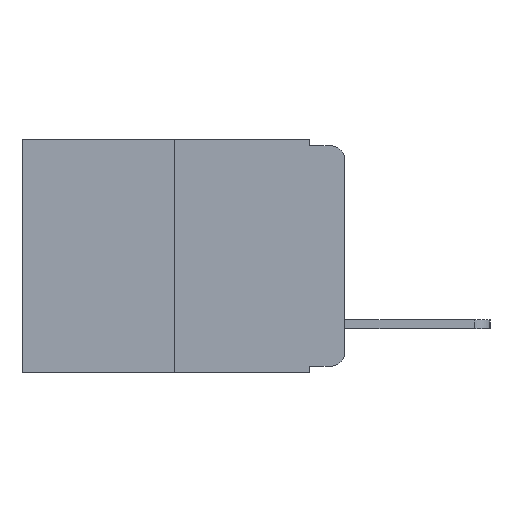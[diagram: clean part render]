
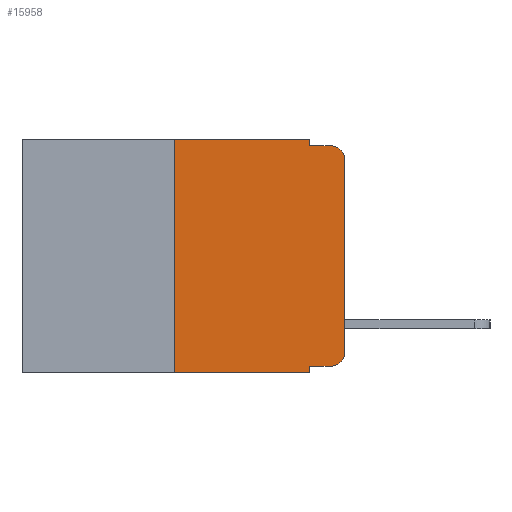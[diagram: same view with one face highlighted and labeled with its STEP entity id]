
A CAD part, left-side view. The second image highlights one B-rep face of the part: STEP entity #15958.
In plain terms, the highlighted planar face has unit normal (-1, 0, 0).
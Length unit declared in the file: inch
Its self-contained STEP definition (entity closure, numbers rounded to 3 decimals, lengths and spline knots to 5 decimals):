
#95 = CARTESIAN_POINT ( 'NONE',  ( 0., 0.25, 0. ) ) ;
#441 = VERTEX_POINT ( 'NONE', #7522 ) ;
#629 = EDGE_CURVE ( 'NONE', #5599, #12527, #10809, .T. ) ;
#1197 = DIRECTION ( 'NONE',  ( 0., -1., 0. ) ) ;
#1220 = VERTEX_POINT ( 'NONE', #19492 ) ;
#1648 = DIRECTION ( 'NONE',  ( 0., 0., -1. ) ) ;
#2439 = VECTOR ( 'NONE', #12449, 39.37008 ) ;
#2592 = CARTESIAN_POINT ( 'NONE',  ( 0., 0.473, 0. ) ) ;
#2681 = VERTEX_POINT ( 'NONE', #3654 ) ;
#2870 = VECTOR ( 'NONE', #18959, 39.37008 ) ;
#2916 = CARTESIAN_POINT ( 'NONE',  ( 0., 0.051, -0.333 ) ) ;
#3638 = CIRCLE ( 'NONE', #15646, 0.02 ) ;
#3654 = CARTESIAN_POINT ( 'NONE',  ( 0., 0.051, -0.333 ) ) ;
#3659 = CARTESIAN_POINT ( 'NONE',  ( 0., 0., 0. ) ) ;
#3790 = DIRECTION ( 'NONE',  ( -1., 0., 0. ) ) ;
#3918 = ORIENTED_EDGE ( 'NONE', *, *, #629, .T. ) ;
#4250 = VECTOR ( 'NONE', #19402, 39.37008 ) ;
#4406 = ORIENTED_EDGE ( 'NONE', *, *, #18420, .T. ) ;
#4427 = EDGE_CURVE ( 'NONE', #5599, #7400, #14295, .T. ) ;
#4751 = CARTESIAN_POINT ( 'NONE',  ( 0., 0.051, -0.01 ) ) ;
#5049 = CARTESIAN_POINT ( 'NONE',  ( 0., 0.473, 0. ) ) ;
#5148 = EDGE_CURVE ( 'NONE', #16173, #11152, #12284, .T. ) ;
#5599 = VERTEX_POINT ( 'NONE', #11612 ) ;
#5987 = CARTESIAN_POINT ( 'NONE',  ( 0., 0.051, 0. ) ) ;
#6458 = VECTOR ( 'NONE', #10842, 39.37008 ) ;
#6759 = VECTOR ( 'NONE', #10499, 39.37008 ) ;
#6897 = LINE ( 'NONE', #2592, #2439 ) ;
#7197 = EDGE_CURVE ( 'NONE', #7400, #18671, #6897, .T. ) ;
#7289 = LINE ( 'NONE', #15903, #2870 ) ;
#7373 = CARTESIAN_POINT ( 'NONE',  ( 0., 0., -0.03 ) ) ;
#7400 = VERTEX_POINT ( 'NONE', #19172 ) ;
#7522 = CARTESIAN_POINT ( 'NONE',  ( 0., 0.02, -0.333 ) ) ;
#7533 = ORIENTED_EDGE ( 'NONE', *, *, #14591, .F. ) ;
#7829 = DIRECTION ( 'NONE',  ( 0., 0., 1. ) ) ;
#8382 = PLANE ( 'NONE',  #8716 ) ;
#8716 = AXIS2_PLACEMENT_3D ( 'NONE', #5049, #11561, #1648 ) ;
#8896 = CARTESIAN_POINT ( 'NONE',  ( 0., 0.051, 0. ) ) ;
#9245 = CARTESIAN_POINT ( 'NONE',  ( 0., 0., -0.313 ) ) ;
#9263 = DIRECTION ( 'NONE',  ( 0., 0., 1. ) ) ;
#9367 = LINE ( 'NONE', #2916, #20849 ) ;
#9461 = CARTESIAN_POINT ( 'NONE',  ( 0., 0.02, -0.313 ) ) ;
#10024 = CARTESIAN_POINT ( 'NONE',  ( 0., 0.051, 0. ) ) ;
#10499 = DIRECTION ( 'NONE',  ( 0., 0., -1. ) ) ;
#10624 = FACE_OUTER_BOUND ( 'NONE', #10813, .T. ) ;
#10809 = LINE ( 'NONE', #17105, #6458 ) ;
#10813 = EDGE_LOOP ( 'NONE', ( #17731, #4406, #10919, #13782, #14993, #13583, #3918, #7533, #17400, #12606 ) ) ;
#10842 = DIRECTION ( 'NONE',  ( 0., -1., 0. ) ) ;
#10919 = ORIENTED_EDGE ( 'NONE', *, *, #17380, .F. ) ;
#11004 = DIRECTION ( 'NONE',  ( 0., 0., -1. ) ) ;
#11014 = EDGE_CURVE ( 'NONE', #18671, #12845, #11101, .T. ) ;
#11101 = LINE ( 'NONE', #8896, #6759 ) ;
#11152 = VERTEX_POINT ( 'NONE', #7373 ) ;
#11405 = EDGE_CURVE ( 'NONE', #441, #16173, #3638, .T. ) ;
#11561 = DIRECTION ( 'NONE',  ( 1., 0., 0. ) ) ;
#11612 = CARTESIAN_POINT ( 'NONE',  ( 0., 0.25, -0.343 ) ) ;
#11808 = VECTOR ( 'NONE', #7829, 39.37008 ) ;
#12284 = LINE ( 'NONE', #3659, #11808 ) ;
#12371 = LINE ( 'NONE', #10024, #4250 ) ;
#12427 = EDGE_CURVE ( 'NONE', #2681, #441, #9367, .T. ) ;
#12449 = DIRECTION ( 'NONE',  ( 0., -1., 0. ) ) ;
#12527 = VERTEX_POINT ( 'NONE', #14508 ) ;
#12606 = ORIENTED_EDGE ( 'NONE', *, *, #11405, .T. ) ;
#12845 = VERTEX_POINT ( 'NONE', #4751 ) ;
#13484 = CARTESIAN_POINT ( 'NONE',  ( 0., 0.02, -0.03 ) ) ;
#13583 = ORIENTED_EDGE ( 'NONE', *, *, #4427, .F. ) ;
#13763 = VECTOR ( 'NONE', #9263, 39.37008 ) ;
#13782 = ORIENTED_EDGE ( 'NONE', *, *, #11014, .F. ) ;
#14295 = LINE ( 'NONE', #95, #13763 ) ;
#14508 = CARTESIAN_POINT ( 'NONE',  ( 0., 0.051, -0.343 ) ) ;
#14591 = EDGE_CURVE ( 'NONE', #2681, #12527, #12371, .T. ) ;
#14993 = ORIENTED_EDGE ( 'NONE', *, *, #7197, .F. ) ;
#15143 = DIRECTION ( 'NONE',  ( 0., 0., -1. ) ) ;
#15646 = AXIS2_PLACEMENT_3D ( 'NONE', #9461, #20406, #11004 ) ;
#15804 = CIRCLE ( 'NONE', #16048, 0.02 ) ;
#15903 = CARTESIAN_POINT ( 'NONE',  ( 0., 0.051, -0.01 ) ) ;
#15958 = ADVANCED_FACE ( 'NONE', ( #10624 ), #8382, .F. ) ;
#16048 = AXIS2_PLACEMENT_3D ( 'NONE', #13484, #3790, #15143 ) ;
#16173 = VERTEX_POINT ( 'NONE', #9245 ) ;
#17105 = CARTESIAN_POINT ( 'NONE',  ( 0., 0.473, -0.343 ) ) ;
#17380 = EDGE_CURVE ( 'NONE', #12845, #1220, #7289, .T. ) ;
#17400 = ORIENTED_EDGE ( 'NONE', *, *, #12427, .T. ) ;
#17731 = ORIENTED_EDGE ( 'NONE', *, *, #5148, .T. ) ;
#18420 = EDGE_CURVE ( 'NONE', #11152, #1220, #15804, .T. ) ;
#18671 = VERTEX_POINT ( 'NONE', #5987 ) ;
#18959 = DIRECTION ( 'NONE',  ( 0., -1., 0. ) ) ;
#19172 = CARTESIAN_POINT ( 'NONE',  ( 0., 0.25, 0. ) ) ;
#19402 = DIRECTION ( 'NONE',  ( 0., 0., -1. ) ) ;
#19492 = CARTESIAN_POINT ( 'NONE',  ( 0., 0.02, -0.01 ) ) ;
#20406 = DIRECTION ( 'NONE',  ( -1., 0., 0. ) ) ;
#20849 = VECTOR ( 'NONE', #1197, 39.37008 ) ;
